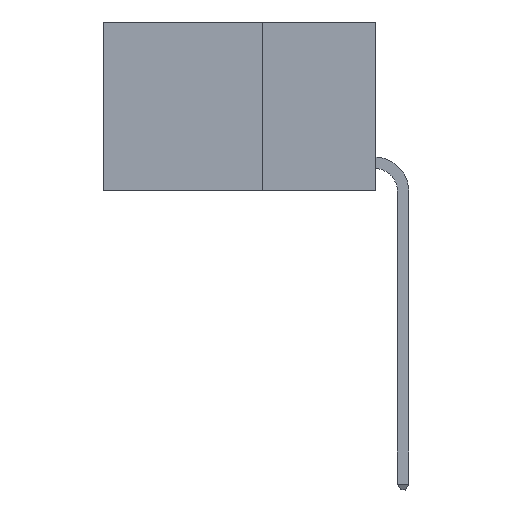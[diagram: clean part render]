
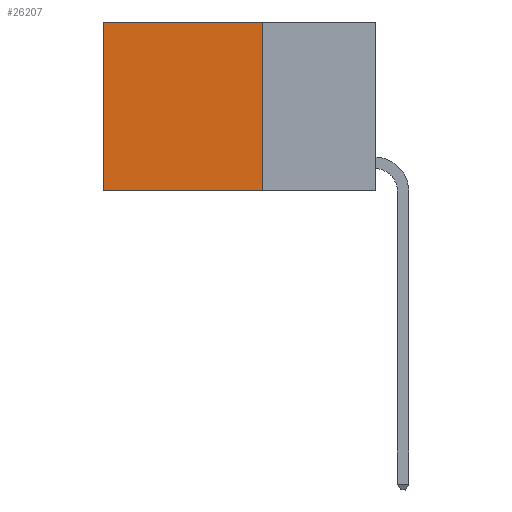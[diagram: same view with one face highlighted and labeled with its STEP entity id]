
A CAD part, left-side view. The second image highlights one B-rep face of the part: STEP entity #26207.
In plain terms, the highlighted planar face has unit normal (-1, 0, 0).
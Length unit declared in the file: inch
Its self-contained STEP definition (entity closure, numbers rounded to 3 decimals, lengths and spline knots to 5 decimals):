
#765 = AXIS2_PLACEMENT_3D ( 'NONE', #15079, #17196, #4817 ) ;
#2665 = CARTESIAN_POINT ( 'NONE',  ( 0.2625, 0.6, 0. ) ) ;
#2703 = PLANE ( 'NONE',  #765 ) ;
#3988 = VECTOR ( 'NONE', #23378, 39.37008 ) ;
#4145 = VECTOR ( 'NONE', #23523, 39.37008 ) ;
#4406 = VECTOR ( 'NONE', #10126, 39.37008 ) ;
#4817 = DIRECTION ( 'NONE',  ( 0., 0., -1. ) ) ;
#4920 = CARTESIAN_POINT ( 'NONE',  ( 0.2625, 0.25, 0. ) ) ;
#6113 = ORIENTED_EDGE ( 'NONE', *, *, #18540, .F. ) ;
#6341 = EDGE_CURVE ( 'NONE', #15606, #10928, #26420, .T. ) ;
#6853 = CARTESIAN_POINT ( 'NONE',  ( 0.2625, 0.25, 0. ) ) ;
#6937 = LINE ( 'NONE', #22868, #12409 ) ;
#9645 = LINE ( 'NONE', #4920, #4145 ) ;
#10126 = DIRECTION ( 'NONE',  ( 0., 1., 0. ) ) ;
#10928 = VERTEX_POINT ( 'NONE', #14278 ) ;
#12149 = ORIENTED_EDGE ( 'NONE', *, *, #6341, .F. ) ;
#12409 = VECTOR ( 'NONE', #16823, 39.37008 ) ;
#12696 = CARTESIAN_POINT ( 'NONE',  ( 0.2625, 0.25, -0.37 ) ) ;
#14278 = CARTESIAN_POINT ( 'NONE',  ( 0.2625, 0.6, -0.37 ) ) ;
#14949 = LINE ( 'NONE', #6853, #3988 ) ;
#14972 = EDGE_CURVE ( 'NONE', #25045, #10928, #6937, .T. ) ;
#15079 = CARTESIAN_POINT ( 'NONE',  ( 0.2625, 0.25, 0. ) ) ;
#15196 = FACE_OUTER_BOUND ( 'NONE', #19691, .T. ) ;
#15606 = VERTEX_POINT ( 'NONE', #12696 ) ;
#15725 = EDGE_CURVE ( 'NONE', #24434, #25045, #14949, .T. ) ;
#16823 = DIRECTION ( 'NONE',  ( 0., 0., -1. ) ) ;
#16878 = ORIENTED_EDGE ( 'NONE', *, *, #15725, .T. ) ;
#17084 = CARTESIAN_POINT ( 'NONE',  ( 0.2625, 0.25, 0. ) ) ;
#17196 = DIRECTION ( 'NONE',  ( 1., 0., 0. ) ) ;
#18540 = EDGE_CURVE ( 'NONE', #24434, #15606, #9645, .T. ) ;
#19691 = EDGE_LOOP ( 'NONE', ( #22330, #12149, #6113, #16878 ) ) ;
#22330 = ORIENTED_EDGE ( 'NONE', *, *, #14972, .T. ) ;
#22868 = CARTESIAN_POINT ( 'NONE',  ( 0.2625, 0.6, 0. ) ) ;
#23378 = DIRECTION ( 'NONE',  ( 0., 1., 0. ) ) ;
#23523 = DIRECTION ( 'NONE',  ( 0., 0., -1. ) ) ;
#24434 = VERTEX_POINT ( 'NONE', #17084 ) ;
#24595 = CARTESIAN_POINT ( 'NONE',  ( 0.2625, 0.25, -0.37 ) ) ;
#25045 = VERTEX_POINT ( 'NONE', #2665 ) ;
#26207 = ADVANCED_FACE ( 'NONE', ( #15196 ), #2703, .F. ) ;
#26420 = LINE ( 'NONE', #24595, #4406 ) ;
